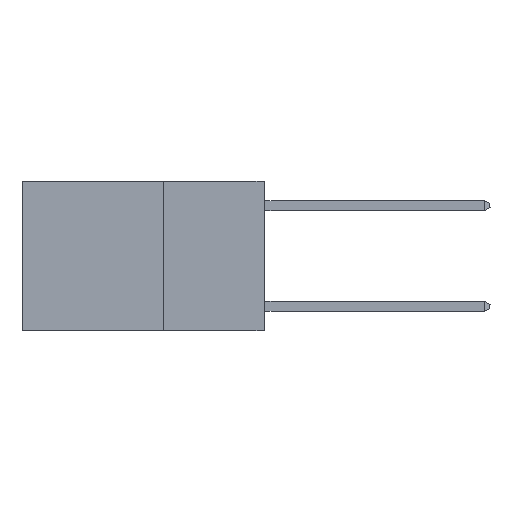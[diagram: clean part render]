
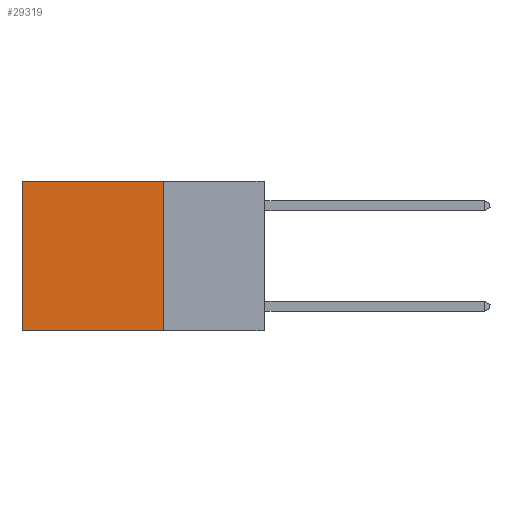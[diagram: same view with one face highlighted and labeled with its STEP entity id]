
A CAD part, left-side view. The second image highlights one B-rep face of the part: STEP entity #29319.
In plain terms, the highlighted planar face has unit normal (-1, 0, 0).
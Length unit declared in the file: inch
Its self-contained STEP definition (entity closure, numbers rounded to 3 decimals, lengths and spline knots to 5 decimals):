
#592 = CARTESIAN_POINT ( 'NONE',  ( 0.2625, 0.6, 0. ) ) ;
#918 = DIRECTION ( 'NONE',  ( 0., 0., -1. ) ) ;
#1841 = LINE ( 'NONE', #21772, #7885 ) ;
#3845 = CARTESIAN_POINT ( 'NONE',  ( 0.2625, 0.25, -0.37 ) ) ;
#3954 = VECTOR ( 'NONE', #7703, 39.37008 ) ;
#4419 = VERTEX_POINT ( 'NONE', #13818 ) ;
#5077 = FACE_OUTER_BOUND ( 'NONE', #18063, .T. ) ;
#5182 = EDGE_CURVE ( 'NONE', #23191, #15294, #1841, .T. ) ;
#5236 = PLANE ( 'NONE',  #6425 ) ;
#6425 = AXIS2_PLACEMENT_3D ( 'NONE', #14874, #17469, #12095 ) ;
#7703 = DIRECTION ( 'NONE',  ( 0., 0., -1. ) ) ;
#7885 = VECTOR ( 'NONE', #31746, 39.37008 ) ;
#8032 = LINE ( 'NONE', #10481, #3954 ) ;
#9365 = CARTESIAN_POINT ( 'NONE',  ( 0.2625, 0.25, 0. ) ) ;
#10369 = LINE ( 'NONE', #592, #31781 ) ;
#10481 = CARTESIAN_POINT ( 'NONE',  ( 0.2625, 0.25, 0. ) ) ;
#10845 = LINE ( 'NONE', #3845, #26973 ) ;
#11117 = ORIENTED_EDGE ( 'NONE', *, *, #11850, .F. ) ;
#11850 = EDGE_CURVE ( 'NONE', #23191, #4419, #8032, .T. ) ;
#12095 = DIRECTION ( 'NONE',  ( 0., 0., -1. ) ) ;
#12799 = VERTEX_POINT ( 'NONE', #27882 ) ;
#12962 = EDGE_CURVE ( 'NONE', #4419, #12799, #10845, .T. ) ;
#13818 = CARTESIAN_POINT ( 'NONE',  ( 0.2625, 0.25, -0.37 ) ) ;
#14874 = CARTESIAN_POINT ( 'NONE',  ( 0.2625, 0.25, 0. ) ) ;
#15294 = VERTEX_POINT ( 'NONE', #19921 ) ;
#17469 = DIRECTION ( 'NONE',  ( 1., 0., 0. ) ) ;
#18063 = EDGE_LOOP ( 'NONE', ( #29919, #26173, #11117, #26069 ) ) ;
#19921 = CARTESIAN_POINT ( 'NONE',  ( 0.2625, 0.6, 0. ) ) ;
#21772 = CARTESIAN_POINT ( 'NONE',  ( 0.2625, 0.25, 0. ) ) ;
#22815 = EDGE_CURVE ( 'NONE', #15294, #12799, #10369, .T. ) ;
#23191 = VERTEX_POINT ( 'NONE', #9365 ) ;
#26069 = ORIENTED_EDGE ( 'NONE', *, *, #5182, .T. ) ;
#26173 = ORIENTED_EDGE ( 'NONE', *, *, #12962, .F. ) ;
#26973 = VECTOR ( 'NONE', #30817, 39.37008 ) ;
#27882 = CARTESIAN_POINT ( 'NONE',  ( 0.2625, 0.6, -0.37 ) ) ;
#29319 = ADVANCED_FACE ( 'NONE', ( #5077 ), #5236, .F. ) ;
#29919 = ORIENTED_EDGE ( 'NONE', *, *, #22815, .T. ) ;
#30817 = DIRECTION ( 'NONE',  ( 0., 1., 0. ) ) ;
#31746 = DIRECTION ( 'NONE',  ( 0., 1., 0. ) ) ;
#31781 = VECTOR ( 'NONE', #918, 39.37008 ) ;
